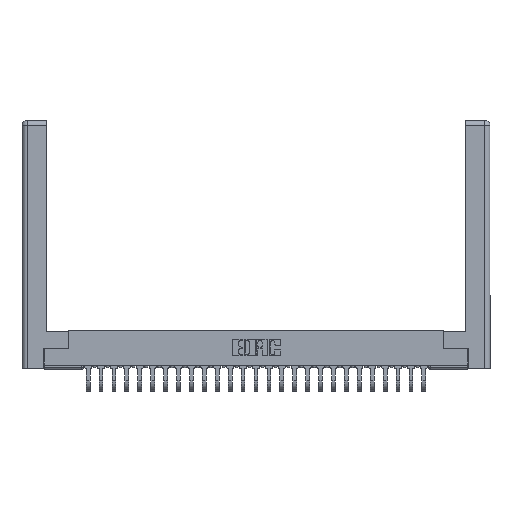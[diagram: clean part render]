
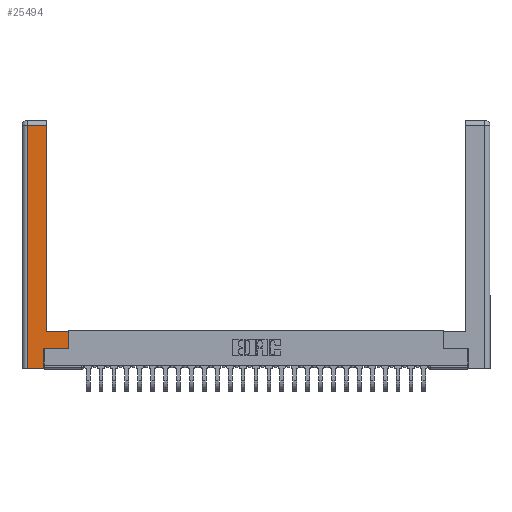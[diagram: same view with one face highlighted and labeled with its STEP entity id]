
A CAD part, top view. The second image highlights one B-rep face of the part: STEP entity #25494.
In plain terms, the highlighted planar face has unit normal (0, 0, 1).
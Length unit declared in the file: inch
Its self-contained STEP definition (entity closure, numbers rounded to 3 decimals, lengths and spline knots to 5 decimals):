
#126 = LINE ( 'NONE', #21418, #11566 ) ;
#478 = LINE ( 'NONE', #11418, #13426 ) ;
#540 = CARTESIAN_POINT ( 'NONE',  ( 0.265, 0., 0. ) ) ;
#804 = CARTESIAN_POINT ( 'NONE',  ( 0.0615, 2.94, 0. ) ) ;
#1171 = LINE ( 'NONE', #20483, #6614 ) ;
#1872 = VECTOR ( 'NONE', #6245, 39.37008 ) ;
#2992 = ORIENTED_EDGE ( 'NONE', *, *, #20623, .T. ) ;
#3044 = ORIENTED_EDGE ( 'NONE', *, *, #10888, .T. ) ;
#3368 = CARTESIAN_POINT ( 'NONE',  ( 0., 0., 0. ) ) ;
#3576 = VECTOR ( 'NONE', #23092, 39.37008 ) ;
#3792 = CARTESIAN_POINT ( 'NONE',  ( 0.295, 2.94, 0. ) ) ;
#3902 = CARTESIAN_POINT ( 'NONE',  ( 0.295, 3., 0. ) ) ;
#3988 = CARTESIAN_POINT ( 'NONE',  ( 0.0615, 0., 0. ) ) ;
#4886 = EDGE_CURVE ( 'NONE', #27470, #18185, #6521, .T. ) ;
#5057 = ORIENTED_EDGE ( 'NONE', *, *, #10167, .T. ) ;
#5088 = DIRECTION ( 'NONE',  ( -1., 0., 0. ) ) ;
#6245 = DIRECTION ( 'NONE',  ( 0., 1., 0. ) ) ;
#6521 = LINE ( 'NONE', #23607, #1872 ) ;
#6533 = ORIENTED_EDGE ( 'NONE', *, *, #11664, .T. ) ;
#6571 = CARTESIAN_POINT ( 'NONE',  ( 0.265, 0.245, 0. ) ) ;
#6614 = VECTOR ( 'NONE', #5088, 39.37008 ) ;
#7294 = EDGE_CURVE ( 'NONE', #11134, #26200, #1171, .T. ) ;
#7349 = CARTESIAN_POINT ( 'NONE',  ( 0.565, 0.245, 0. ) ) ;
#7431 = CARTESIAN_POINT ( 'NONE',  ( 0.0615, 2.94, 0. ) ) ;
#7797 = ORIENTED_EDGE ( 'NONE', *, *, #19140, .T. ) ;
#7857 = VERTEX_POINT ( 'NONE', #3792 ) ;
#8930 = LINE ( 'NONE', #17321, #24208 ) ;
#8946 = DIRECTION ( 'NONE',  ( 0., -1., 0. ) ) ;
#8949 = LINE ( 'NONE', #540, #17508 ) ;
#10167 = EDGE_CURVE ( 'NONE', #7857, #27717, #26665, .T. ) ;
#10852 = CARTESIAN_POINT ( 'NONE',  ( 0.295, 0.45, 0. ) ) ;
#10888 = EDGE_CURVE ( 'NONE', #18185, #17440, #478, .T. ) ;
#11134 = VERTEX_POINT ( 'NONE', #12891 ) ;
#11418 = CARTESIAN_POINT ( 'NONE',  ( 0.565, 0.245, 0. ) ) ;
#11566 = VECTOR ( 'NONE', #8946, 39.37008 ) ;
#11664 = EDGE_CURVE ( 'NONE', #17440, #11134, #8930, .T. ) ;
#11906 = DIRECTION ( 'NONE',  ( -1., 0., 0. ) ) ;
#12891 = CARTESIAN_POINT ( 'NONE',  ( 0.565, 0.45, 0. ) ) ;
#13107 = AXIS2_PLACEMENT_3D ( 'NONE', #3368, #24520, #11906 ) ;
#13110 = DIRECTION ( 'NONE',  ( 1., 0., 0. ) ) ;
#13426 = VECTOR ( 'NONE', #13110, 39.37008 ) ;
#15839 = VERTEX_POINT ( 'NONE', #3988 ) ;
#15966 = DIRECTION ( 'NONE',  ( -1., 0., 0. ) ) ;
#16826 = ORIENTED_EDGE ( 'NONE', *, *, #7294, .T. ) ;
#17214 = DIRECTION ( 'NONE',  ( 1., 0., 0. ) ) ;
#17321 = CARTESIAN_POINT ( 'NONE',  ( 0.565, 0.45, 0. ) ) ;
#17440 = VERTEX_POINT ( 'NONE', #7349 ) ;
#17508 = VECTOR ( 'NONE', #17214, 39.37008 ) ;
#18154 = EDGE_CURVE ( 'NONE', #15839, #27470, #8949, .T. ) ;
#18185 = VERTEX_POINT ( 'NONE', #6571 ) ;
#19140 = EDGE_CURVE ( 'NONE', #27717, #15839, #126, .T. ) ;
#20310 = EDGE_LOOP ( 'NONE', ( #2992, #5057, #7797, #24618, #21446, #3044, #6533, #16826 ) ) ;
#20483 = CARTESIAN_POINT ( 'NONE',  ( 0.295, 0.45, 0. ) ) ;
#20623 = EDGE_CURVE ( 'NONE', #26200, #7857, #20848, .T. ) ;
#20848 = LINE ( 'NONE', #3902, #3576 ) ;
#21418 = CARTESIAN_POINT ( 'NONE',  ( 0.0615, 0., 0. ) ) ;
#21446 = ORIENTED_EDGE ( 'NONE', *, *, #4886, .T. ) ;
#22684 = FACE_OUTER_BOUND ( 'NONE', #20310, .T. ) ;
#23092 = DIRECTION ( 'NONE',  ( 0., 1., 0. ) ) ;
#23607 = CARTESIAN_POINT ( 'NONE',  ( 0.265, 0.245, 0. ) ) ;
#24208 = VECTOR ( 'NONE', #25917, 39.37008 ) ;
#24520 = DIRECTION ( 'NONE',  ( 0., 0., -1. ) ) ;
#24618 = ORIENTED_EDGE ( 'NONE', *, *, #18154, .T. ) ;
#25095 = CARTESIAN_POINT ( 'NONE',  ( 0.265, 0., 0. ) ) ;
#25494 = ADVANCED_FACE ( 'NONE', ( #22684 ), #26658, .F. ) ;
#25917 = DIRECTION ( 'NONE',  ( 0., 1., 0. ) ) ;
#26200 = VERTEX_POINT ( 'NONE', #10852 ) ;
#26658 = PLANE ( 'NONE',  #13107 ) ;
#26665 = LINE ( 'NONE', #7431, #27303 ) ;
#27303 = VECTOR ( 'NONE', #15966, 39.37008 ) ;
#27470 = VERTEX_POINT ( 'NONE', #25095 ) ;
#27717 = VERTEX_POINT ( 'NONE', #804 ) ;
